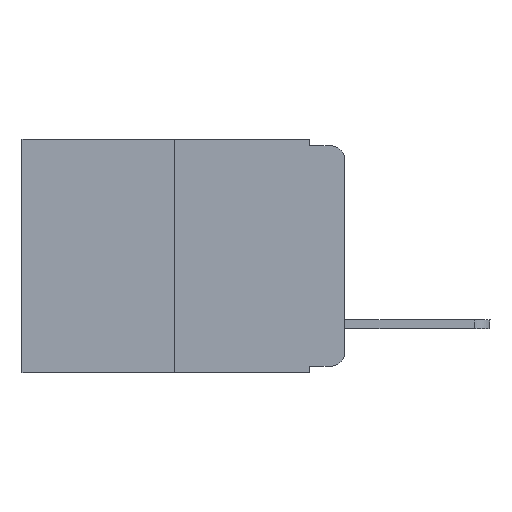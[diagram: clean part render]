
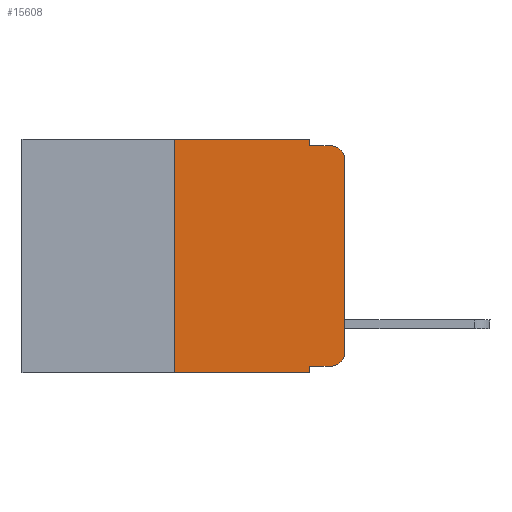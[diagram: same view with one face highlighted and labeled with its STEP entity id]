
A CAD part, left-side view. The second image highlights one B-rep face of the part: STEP entity #15608.
In plain terms, the highlighted planar face has unit normal (-1, 0, 0).
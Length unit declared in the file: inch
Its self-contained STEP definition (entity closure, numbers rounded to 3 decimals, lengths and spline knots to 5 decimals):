
#7 = VERTEX_POINT ( 'NONE', #3172 ) ;
#103 = VERTEX_POINT ( 'NONE', #1962 ) ;
#439 = VERTEX_POINT ( 'NONE', #756 ) ;
#519 = CARTESIAN_POINT ( 'NONE',  ( 0., 0.02, -0.01 ) ) ;
#726 = CIRCLE ( 'NONE', #13775, 0.02 ) ;
#756 = CARTESIAN_POINT ( 'NONE',  ( 0., 0.02, -0.333 ) ) ;
#970 = DIRECTION ( 'NONE',  ( 0., 0., -1. ) ) ;
#1039 = DIRECTION ( 'NONE',  ( 1., 0., 0. ) ) ;
#1221 = VERTEX_POINT ( 'NONE', #1291 ) ;
#1291 = CARTESIAN_POINT ( 'NONE',  ( 0., 0.051, -0.333 ) ) ;
#1305 = CARTESIAN_POINT ( 'NONE',  ( 0., 0., -0.313 ) ) ;
#1392 = CARTESIAN_POINT ( 'NONE',  ( 0., 0.473, -0.343 ) ) ;
#1577 = VECTOR ( 'NONE', #13351, 39.37008 ) ;
#1700 = VERTEX_POINT ( 'NONE', #1305 ) ;
#1962 = CARTESIAN_POINT ( 'NONE',  ( 0., 0., -0.03 ) ) ;
#1981 = ORIENTED_EDGE ( 'NONE', *, *, #9399, .F. ) ;
#2119 = CARTESIAN_POINT ( 'NONE',  ( 0., 0.25, 0. ) ) ;
#2471 = AXIS2_PLACEMENT_3D ( 'NONE', #5456, #12589, #12663 ) ;
#2751 = ORIENTED_EDGE ( 'NONE', *, *, #10093, .F. ) ;
#3172 = CARTESIAN_POINT ( 'NONE',  ( 0., 0.25, -0.343 ) ) ;
#3345 = EDGE_CURVE ( 'NONE', #1221, #439, #7106, .T. ) ;
#3980 = VERTEX_POINT ( 'NONE', #519 ) ;
#4420 = EDGE_CURVE ( 'NONE', #5652, #10342, #15164, .T. ) ;
#4475 = LINE ( 'NONE', #15538, #7906 ) ;
#4699 = DIRECTION ( 'NONE',  ( 0., 0., -1. ) ) ;
#4897 = EDGE_CURVE ( 'NONE', #1221, #9192, #14247, .T. ) ;
#5456 = CARTESIAN_POINT ( 'NONE',  ( 0., 0.02, -0.313 ) ) ;
#5652 = VERTEX_POINT ( 'NONE', #2119 ) ;
#5708 = EDGE_CURVE ( 'NONE', #7, #9192, #13466, .T. ) ;
#5728 = CARTESIAN_POINT ( 'NONE',  ( 0., 0.051, 0. ) ) ;
#5983 = LINE ( 'NONE', #11182, #6602 ) ;
#6068 = CARTESIAN_POINT ( 'NONE',  ( 0., 0.02, -0.03 ) ) ;
#6233 = ORIENTED_EDGE ( 'NONE', *, *, #5708, .T. ) ;
#6262 = DIRECTION ( 'NONE',  ( 0., -1., 0. ) ) ;
#6544 = VECTOR ( 'NONE', #6262, 39.37008 ) ;
#6602 = VECTOR ( 'NONE', #12221, 39.37008 ) ;
#6634 = CARTESIAN_POINT ( 'NONE',  ( 0., 0.051, 0. ) ) ;
#6934 = LINE ( 'NONE', #8280, #14606 ) ;
#7010 = EDGE_CURVE ( 'NONE', #439, #1700, #12442, .T. ) ;
#7106 = LINE ( 'NONE', #11993, #7476 ) ;
#7134 = ORIENTED_EDGE ( 'NONE', *, *, #7010, .T. ) ;
#7255 = LINE ( 'NONE', #12140, #1577 ) ;
#7476 = VECTOR ( 'NONE', #15847, 39.37008 ) ;
#7849 = VERTEX_POINT ( 'NONE', #11738 ) ;
#7906 = VECTOR ( 'NONE', #970, 39.37008 ) ;
#8078 = FACE_OUTER_BOUND ( 'NONE', #9441, .T. ) ;
#8280 = CARTESIAN_POINT ( 'NONE',  ( 0., 0., 0. ) ) ;
#8476 = AXIS2_PLACEMENT_3D ( 'NONE', #15698, #1039, #4699 ) ;
#8877 = ORIENTED_EDGE ( 'NONE', *, *, #14738, .T. ) ;
#9192 = VERTEX_POINT ( 'NONE', #11842 ) ;
#9399 = EDGE_CURVE ( 'NONE', #7849, #3980, #5983, .T. ) ;
#9412 = DIRECTION ( 'NONE',  ( 0., 0., 1. ) ) ;
#9441 = EDGE_LOOP ( 'NONE', ( #8877, #14887, #1981, #2751, #11218, #12041, #6233, #10686, #14714, #7134 ) ) ;
#10093 = EDGE_CURVE ( 'NONE', #10342, #7849, #4475, .T. ) ;
#10342 = VERTEX_POINT ( 'NONE', #6634 ) ;
#10570 = VECTOR ( 'NONE', #15084, 39.37008 ) ;
#10637 = PLANE ( 'NONE',  #8476 ) ;
#10686 = ORIENTED_EDGE ( 'NONE', *, *, #4897, .F. ) ;
#10969 = DIRECTION ( 'NONE',  ( -1., 0., 0. ) ) ;
#11182 = CARTESIAN_POINT ( 'NONE',  ( 0., 0.051, -0.01 ) ) ;
#11218 = ORIENTED_EDGE ( 'NONE', *, *, #4420, .F. ) ;
#11738 = CARTESIAN_POINT ( 'NONE',  ( 0., 0.051, -0.01 ) ) ;
#11842 = CARTESIAN_POINT ( 'NONE',  ( 0., 0.051, -0.343 ) ) ;
#11993 = CARTESIAN_POINT ( 'NONE',  ( 0., 0.051, -0.333 ) ) ;
#12041 = ORIENTED_EDGE ( 'NONE', *, *, #15671, .F. ) ;
#12140 = CARTESIAN_POINT ( 'NONE',  ( 0., 0.25, 0. ) ) ;
#12221 = DIRECTION ( 'NONE',  ( 0., -1., 0. ) ) ;
#12442 = CIRCLE ( 'NONE', #2471, 0.02 ) ;
#12589 = DIRECTION ( 'NONE',  ( -1., 0., 0. ) ) ;
#12642 = EDGE_CURVE ( 'NONE', #103, #3980, #726, .T. ) ;
#12663 = DIRECTION ( 'NONE',  ( 0., 0., -1. ) ) ;
#13048 = DIRECTION ( 'NONE',  ( 0., 0., -1. ) ) ;
#13351 = DIRECTION ( 'NONE',  ( 0., 0., 1. ) ) ;
#13466 = LINE ( 'NONE', #1392, #6544 ) ;
#13775 = AXIS2_PLACEMENT_3D ( 'NONE', #6068, #10969, #13048 ) ;
#14044 = CARTESIAN_POINT ( 'NONE',  ( 0., 0.473, 0. ) ) ;
#14247 = LINE ( 'NONE', #5728, #14380 ) ;
#14380 = VECTOR ( 'NONE', #15271, 39.37008 ) ;
#14606 = VECTOR ( 'NONE', #9412, 39.37008 ) ;
#14714 = ORIENTED_EDGE ( 'NONE', *, *, #3345, .T. ) ;
#14738 = EDGE_CURVE ( 'NONE', #1700, #103, #6934, .T. ) ;
#14887 = ORIENTED_EDGE ( 'NONE', *, *, #12642, .T. ) ;
#15084 = DIRECTION ( 'NONE',  ( 0., -1., 0. ) ) ;
#15164 = LINE ( 'NONE', #14044, #10570 ) ;
#15271 = DIRECTION ( 'NONE',  ( 0., 0., -1. ) ) ;
#15538 = CARTESIAN_POINT ( 'NONE',  ( 0., 0.051, 0. ) ) ;
#15608 = ADVANCED_FACE ( 'NONE', ( #8078 ), #10637, .F. ) ;
#15671 = EDGE_CURVE ( 'NONE', #7, #5652, #7255, .T. ) ;
#15698 = CARTESIAN_POINT ( 'NONE',  ( 0., 0.473, 0. ) ) ;
#15847 = DIRECTION ( 'NONE',  ( 0., -1., 0. ) ) ;
